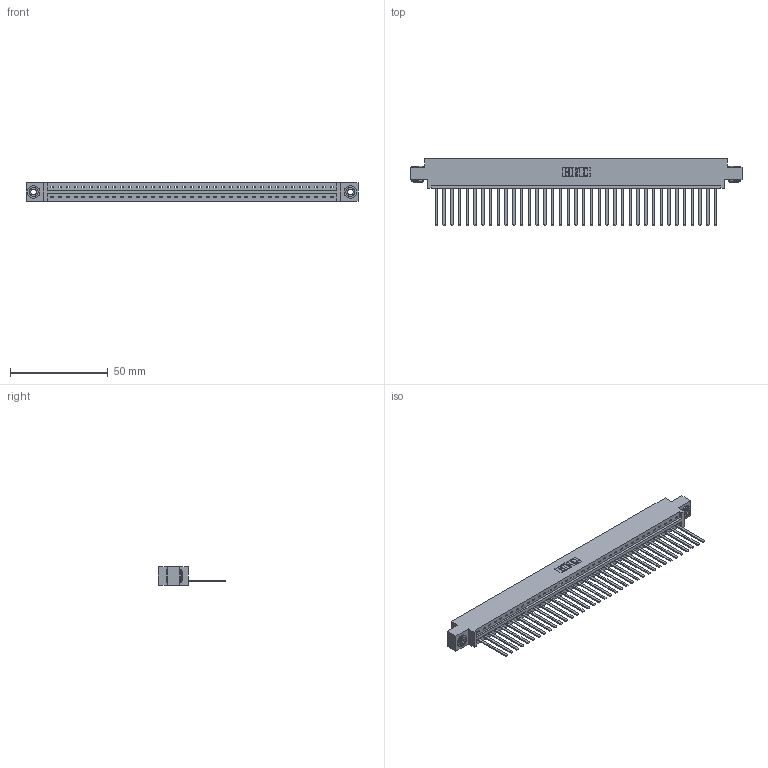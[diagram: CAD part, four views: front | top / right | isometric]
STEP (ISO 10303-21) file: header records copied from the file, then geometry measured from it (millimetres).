
FILE_DESCRIPTION (( 'STEP AP203' ), '1' );
FILE_NAME ('387-037-544-603.STEP', '2018-09-19T03:12:14', ( '' ), ( '' ), 'SwSTEP 2.0', 'SolidWorks 2016', '' );
FILE_SCHEMA (( 'CONFIG_CONTROL_DESIGN' ));
Length unit declared in the file: inch
Products named in the file (4): 337 Part_0.170 Offset - 0.156 Dia-TH; 345-292-001_345-293-144; 345-250-002_345-250-002-102; 387-037-544-603
Assembly tree (40 placements, depth 2):
  387-037-544-603
    337 Part_0.170 Offset - 0.156 Dia-TH
    345-292-001_345-293-144  x37
    345-250-002_345-250-002-102  x2
Bounding box: 169.62 x 34.3 x 9.4 mm (x, y, z)
Volume: 17897.1 mm3; surface area: 20205 mm2
Topology: 40 solids, 40 shells, 2228 faces, 6689 edges, 4406 vertices
Faces by surface type: plane 1638, cylinder 582, cone 8
Entity records: 28748 total; most frequent: CARTESIAN_POINT 4984, ORIENTED_EDGE 4950, DIRECTION 4235, EDGE_CURVE 2475, LINE 2327, VECTOR 2327, VERTEX_POINT 1646, AXIS2_PLACEMENT_3D 954
